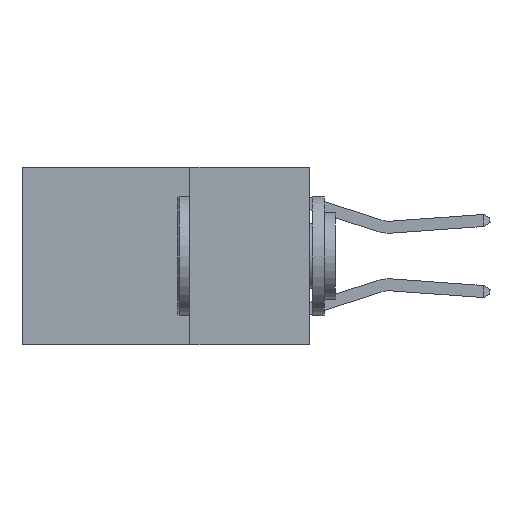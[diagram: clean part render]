
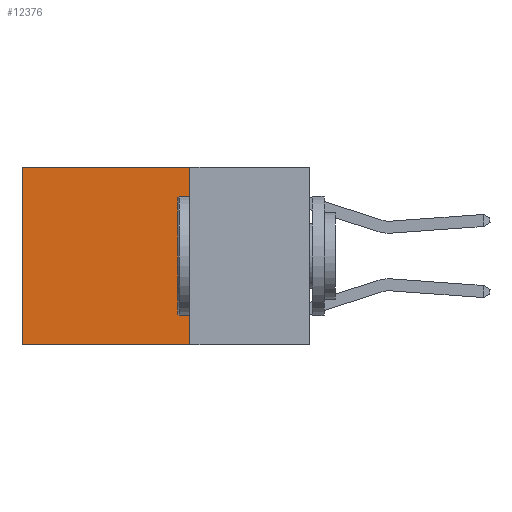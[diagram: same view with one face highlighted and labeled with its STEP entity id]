
A CAD part, left-side view. The second image highlights one B-rep face of the part: STEP entity #12376.
In plain terms, the highlighted planar face has unit normal (-1, 0, 0).
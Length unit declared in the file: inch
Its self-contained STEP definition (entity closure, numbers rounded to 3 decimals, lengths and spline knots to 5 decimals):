
#1 = CARTESIAN_POINT ( 'NONE',  ( 0.2625, 0.25, 0. ) ) ;
#1065 = EDGE_CURVE ( 'NONE', #21158, #25961, #9568, .T. ) ;
#1753 = VECTOR ( 'NONE', #23103, 39.37008 ) ;
#2085 = VECTOR ( 'NONE', #21925, 39.37008 ) ;
#2516 = EDGE_CURVE ( 'NONE', #4513, #4164, #14718, .T. ) ;
#2642 = EDGE_CURVE ( 'NONE', #21158, #4513, #22978, .T. ) ;
#2961 = CARTESIAN_POINT ( 'NONE',  ( 0.2625, 0.25, 0. ) ) ;
#4164 = VERTEX_POINT ( 'NONE', #15776 ) ;
#4513 = VERTEX_POINT ( 'NONE', #13231 ) ;
#5670 = LINE ( 'NONE', #7917, #25034 ) ;
#5721 = EDGE_LOOP ( 'NONE', ( #15583, #24995, #21016, #7482 ) ) ;
#6466 = CARTESIAN_POINT ( 'NONE',  ( 0.2625, 0.25, 0. ) ) ;
#6576 = EDGE_CURVE ( 'NONE', #25961, #4164, #5670, .T. ) ;
#7482 = ORIENTED_EDGE ( 'NONE', *, *, #1065, .T. ) ;
#7917 = CARTESIAN_POINT ( 'NONE',  ( 0.2625, 0.6, 0. ) ) ;
#8058 = FACE_OUTER_BOUND ( 'NONE', #5721, .T. ) ;
#8194 = DIRECTION ( 'NONE',  ( 0., 0., -1. ) ) ;
#9332 = VECTOR ( 'NONE', #16937, 39.37008 ) ;
#9568 = LINE ( 'NONE', #25766, #2085 ) ;
#11013 = AXIS2_PLACEMENT_3D ( 'NONE', #1, #13981, #8194 ) ;
#12133 = CARTESIAN_POINT ( 'NONE',  ( 0.2625, 0.6, 0. ) ) ;
#12376 = ADVANCED_FACE ( 'NONE', ( #8058 ), #23979, .F. ) ;
#13231 = CARTESIAN_POINT ( 'NONE',  ( 0.2625, 0.25, -0.37 ) ) ;
#13981 = DIRECTION ( 'NONE',  ( 1., 0., 0. ) ) ;
#14718 = LINE ( 'NONE', #22322, #9332 ) ;
#15583 = ORIENTED_EDGE ( 'NONE', *, *, #6576, .T. ) ;
#15776 = CARTESIAN_POINT ( 'NONE',  ( 0.2625, 0.6, -0.37 ) ) ;
#16937 = DIRECTION ( 'NONE',  ( 0., 1., 0. ) ) ;
#21016 = ORIENTED_EDGE ( 'NONE', *, *, #2642, .F. ) ;
#21158 = VERTEX_POINT ( 'NONE', #6466 ) ;
#21925 = DIRECTION ( 'NONE',  ( 0., 1., 0. ) ) ;
#22322 = CARTESIAN_POINT ( 'NONE',  ( 0.2625, 0.25, -0.37 ) ) ;
#22978 = LINE ( 'NONE', #2961, #1753 ) ;
#23103 = DIRECTION ( 'NONE',  ( 0., 0., -1. ) ) ;
#23979 = PLANE ( 'NONE',  #11013 ) ;
#24995 = ORIENTED_EDGE ( 'NONE', *, *, #2516, .F. ) ;
#25034 = VECTOR ( 'NONE', #25679, 39.37008 ) ;
#25679 = DIRECTION ( 'NONE',  ( 0., 0., -1. ) ) ;
#25766 = CARTESIAN_POINT ( 'NONE',  ( 0.2625, 0.25, 0. ) ) ;
#25961 = VERTEX_POINT ( 'NONE', #12133 ) ;
